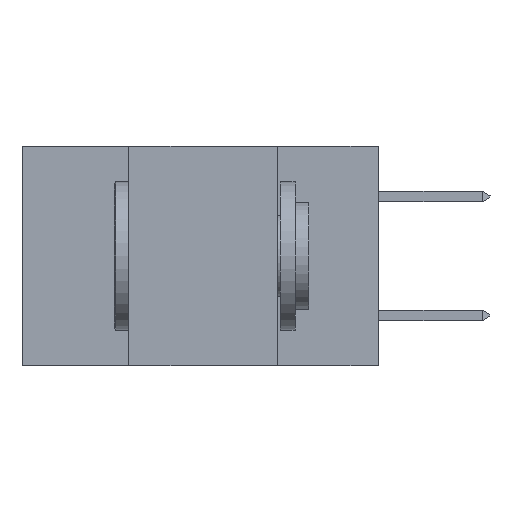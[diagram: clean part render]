
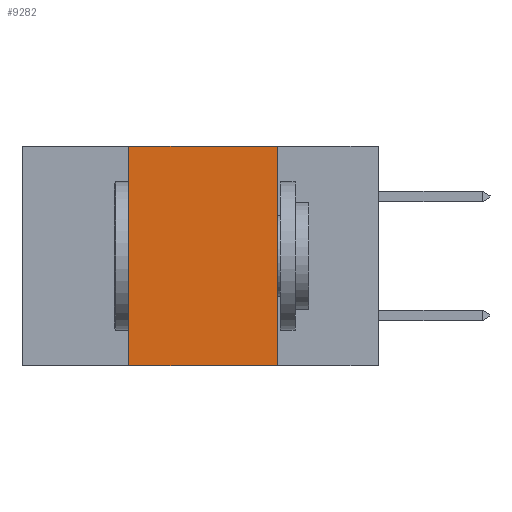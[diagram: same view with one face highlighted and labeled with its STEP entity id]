
A CAD part, left-side view. The second image highlights one B-rep face of the part: STEP entity #9282.
In plain terms, the highlighted planar face has unit normal (-1, 0, 0).
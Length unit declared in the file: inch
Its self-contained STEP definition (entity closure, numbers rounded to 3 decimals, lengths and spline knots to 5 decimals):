
#316 = LINE ( 'NONE', #11909, #9456 ) ;
#730 = ORIENTED_EDGE ( 'NONE', *, *, #15914, .F. ) ;
#1057 = ORIENTED_EDGE ( 'NONE', *, *, #3474, .F. ) ;
#1683 = CARTESIAN_POINT ( 'NONE',  ( 0., 0.42, 0. ) ) ;
#1704 = CARTESIAN_POINT ( 'NONE',  ( 0., 0.6, -0.37 ) ) ;
#2914 = PLANE ( 'NONE',  #15587 ) ;
#3229 = VERTEX_POINT ( 'NONE', #1683 ) ;
#3474 = EDGE_CURVE ( 'NONE', #18062, #3229, #15313, .T. ) ;
#4337 = FACE_OUTER_BOUND ( 'NONE', #16267, .T. ) ;
#4690 = VECTOR ( 'NONE', #7516, 39.37008 ) ;
#5168 = DIRECTION ( 'NONE',  ( 0., 0., 1. ) ) ;
#5278 = CARTESIAN_POINT ( 'NONE',  ( 0., 0.42, -0.37 ) ) ;
#6055 = VERTEX_POINT ( 'NONE', #10633 ) ;
#6261 = LINE ( 'NONE', #1704, #4690 ) ;
#6556 = CARTESIAN_POINT ( 'NONE',  ( 0., 0.17, -0.37 ) ) ;
#7516 = DIRECTION ( 'NONE',  ( 0., -1., 0. ) ) ;
#8179 = VERTEX_POINT ( 'NONE', #15284 ) ;
#8527 = DIRECTION ( 'NONE',  ( 1., 0., 0. ) ) ;
#8976 = EDGE_CURVE ( 'NONE', #18062, #8179, #6261, .T. ) ;
#9282 = ADVANCED_FACE ( 'NONE', ( #4337 ), #2914, .F. ) ;
#9456 = VECTOR ( 'NONE', #17660, 39.37008 ) ;
#10466 = CARTESIAN_POINT ( 'NONE',  ( 0., 0.42, -0.37 ) ) ;
#10633 = CARTESIAN_POINT ( 'NONE',  ( 0., 0.17, 0. ) ) ;
#11481 = VECTOR ( 'NONE', #16003, 39.37008 ) ;
#11626 = EDGE_CURVE ( 'NONE', #6055, #8179, #12992, .T. ) ;
#11909 = CARTESIAN_POINT ( 'NONE',  ( 0., 0.6, 0. ) ) ;
#12992 = LINE ( 'NONE', #6556, #11481 ) ;
#15284 = CARTESIAN_POINT ( 'NONE',  ( 0., 0.17, -0.37 ) ) ;
#15313 = LINE ( 'NONE', #5278, #17496 ) ;
#15587 = AXIS2_PLACEMENT_3D ( 'NONE', #17210, #8527, #15798 ) ;
#15798 = DIRECTION ( 'NONE',  ( 0., 0., -1. ) ) ;
#15914 = EDGE_CURVE ( 'NONE', #3229, #6055, #316, .T. ) ;
#16003 = DIRECTION ( 'NONE',  ( 0., 0., -1. ) ) ;
#16267 = EDGE_LOOP ( 'NONE', ( #18442, #730, #1057, #16932 ) ) ;
#16932 = ORIENTED_EDGE ( 'NONE', *, *, #8976, .T. ) ;
#17210 = CARTESIAN_POINT ( 'NONE',  ( 0., 0.6, 0. ) ) ;
#17496 = VECTOR ( 'NONE', #5168, 39.37008 ) ;
#17660 = DIRECTION ( 'NONE',  ( 0., -1., 0. ) ) ;
#18062 = VERTEX_POINT ( 'NONE', #10466 ) ;
#18442 = ORIENTED_EDGE ( 'NONE', *, *, #11626, .F. ) ;
